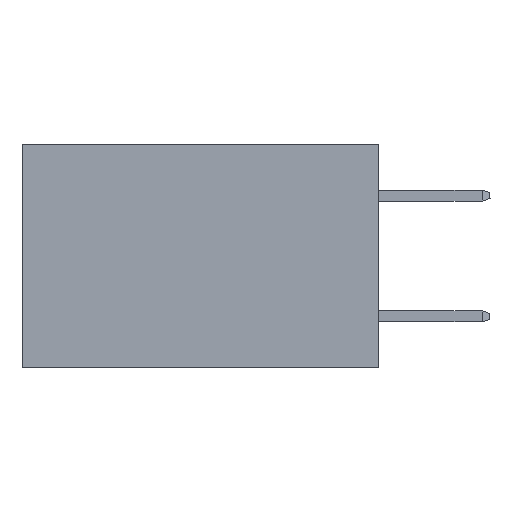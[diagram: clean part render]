
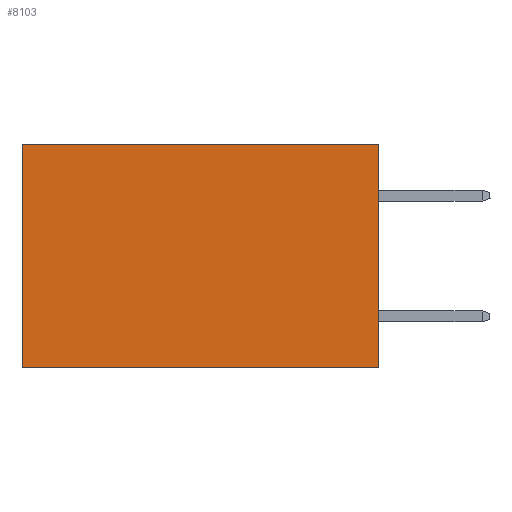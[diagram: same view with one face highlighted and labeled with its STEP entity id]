
A CAD part, left-side view. The second image highlights one B-rep face of the part: STEP entity #8103.
In plain terms, the highlighted planar face has unit normal (-1, 0, 0).
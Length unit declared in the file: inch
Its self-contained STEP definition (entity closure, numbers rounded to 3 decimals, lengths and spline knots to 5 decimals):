
#3711 = CARTESIAN_POINT ( 'NONE',  ( 0.277, 0.59, -0.37 ) ) ;
#4013 = ORIENTED_EDGE ( 'NONE', *, *, #25787, .T. ) ;
#4855 = DIRECTION ( 'NONE',  ( 0., 0., -1. ) ) ;
#5328 = CARTESIAN_POINT ( 'NONE',  ( 0.277, 0., 0. ) ) ;
#6076 = FACE_OUTER_BOUND ( 'NONE', #21802, .T. ) ;
#6578 = DIRECTION ( 'NONE',  ( 1., 0., 0. ) ) ;
#8103 = ADVANCED_FACE ( 'NONE', ( #6076 ), #19364, .F. ) ;
#9334 = ORIENTED_EDGE ( 'NONE', *, *, #31606, .F. ) ;
#9771 = VECTOR ( 'NONE', #4855, 39.37008 ) ;
#10303 = VERTEX_POINT ( 'NONE', #22172 ) ;
#10567 = LINE ( 'NONE', #30497, #9771 ) ;
#12562 = LINE ( 'NONE', #14420, #18613 ) ;
#13038 = VERTEX_POINT ( 'NONE', #20714 ) ;
#13775 = AXIS2_PLACEMENT_3D ( 'NONE', #19252, #6578, #24566 ) ;
#14420 = CARTESIAN_POINT ( 'NONE',  ( 0.277, 0., -0.37 ) ) ;
#15006 = ORIENTED_EDGE ( 'NONE', *, *, #21116, .T. ) ;
#17005 = DIRECTION ( 'NONE',  ( 0., 1., 0. ) ) ;
#17625 = VERTEX_POINT ( 'NONE', #5328 ) ;
#17899 = VECTOR ( 'NONE', #23211, 39.37008 ) ;
#18051 = CARTESIAN_POINT ( 'NONE',  ( 0.277, 0., 0. ) ) ;
#18613 = VECTOR ( 'NONE', #17005, 39.37008 ) ;
#19252 = CARTESIAN_POINT ( 'NONE',  ( 0.277, 0., -0.37 ) ) ;
#19364 = PLANE ( 'NONE',  #13775 ) ;
#19600 = CARTESIAN_POINT ( 'NONE',  ( 0.277, 0., -0.37 ) ) ;
#20403 = VECTOR ( 'NONE', #29975, 39.37008 ) ;
#20714 = CARTESIAN_POINT ( 'NONE',  ( 0.277, 0.59, 0. ) ) ;
#21116 = EDGE_CURVE ( 'NONE', #17625, #13038, #30788, .T. ) ;
#21802 = EDGE_LOOP ( 'NONE', ( #4013, #24912, #9334, #15006 ) ) ;
#21981 = EDGE_CURVE ( 'NONE', #10303, #28241, #12562, .T. ) ;
#22172 = CARTESIAN_POINT ( 'NONE',  ( 0.277, 0., -0.37 ) ) ;
#23211 = DIRECTION ( 'NONE',  ( 0., 1., 0. ) ) ;
#24566 = DIRECTION ( 'NONE',  ( 0., 0., -1. ) ) ;
#24912 = ORIENTED_EDGE ( 'NONE', *, *, #21981, .F. ) ;
#25787 = EDGE_CURVE ( 'NONE', #13038, #28241, #10567, .T. ) ;
#28104 = LINE ( 'NONE', #19600, #20403 ) ;
#28241 = VERTEX_POINT ( 'NONE', #3711 ) ;
#29975 = DIRECTION ( 'NONE',  ( 0., 0., -1. ) ) ;
#30497 = CARTESIAN_POINT ( 'NONE',  ( 0.277, 0.59, -0.37 ) ) ;
#30788 = LINE ( 'NONE', #18051, #17899 ) ;
#31606 = EDGE_CURVE ( 'NONE', #17625, #10303, #28104, .T. ) ;
